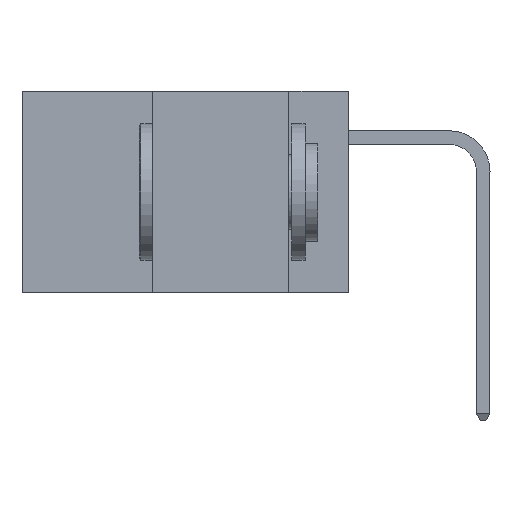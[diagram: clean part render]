
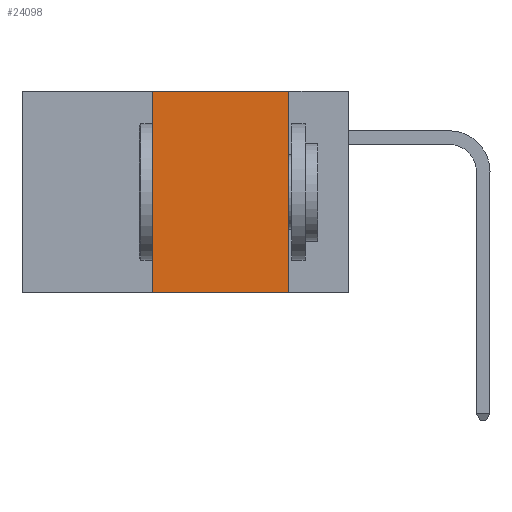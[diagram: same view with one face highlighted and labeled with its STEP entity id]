
A CAD part, left-side view. The second image highlights one B-rep face of the part: STEP entity #24098.
In plain terms, the highlighted planar face has unit normal (-1, 0, 0).
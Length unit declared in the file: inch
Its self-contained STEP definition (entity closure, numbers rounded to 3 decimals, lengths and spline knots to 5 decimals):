
#1826 = EDGE_CURVE ( 'NONE', #2224, #15288, #28103, .T. ) ;
#2224 = VERTEX_POINT ( 'NONE', #34427 ) ;
#2913 = VECTOR ( 'NONE', #7271, 39.37008 ) ;
#3601 = CARTESIAN_POINT ( 'NONE',  ( 0., 0.36, 0. ) ) ;
#5559 = EDGE_LOOP ( 'NONE', ( #30382, #32151, #26294, #21564 ) ) ;
#6026 = DIRECTION ( 'NONE',  ( 0., 0., -1. ) ) ;
#7073 = LINE ( 'NONE', #3601, #22240 ) ;
#7271 = DIRECTION ( 'NONE',  ( 0., -1., 0. ) ) ;
#11660 = LINE ( 'NONE', #21625, #2913 ) ;
#12340 = DIRECTION ( 'NONE',  ( 0., 0., 1. ) ) ;
#12544 = EDGE_CURVE ( 'NONE', #22524, #2224, #23413, .T. ) ;
#13331 = AXIS2_PLACEMENT_3D ( 'NONE', #20312, #23101, #6026 ) ;
#15288 = VERTEX_POINT ( 'NONE', #19332 ) ;
#16346 = EDGE_CURVE ( 'NONE', #26613, #15288, #11660, .T. ) ;
#18051 = DIRECTION ( 'NONE',  ( 0., -1., 0. ) ) ;
#19332 = CARTESIAN_POINT ( 'NONE',  ( 0., 0.11, -0.37 ) ) ;
#20312 = CARTESIAN_POINT ( 'NONE',  ( 0., 0.6, 0. ) ) ;
#21564 = ORIENTED_EDGE ( 'NONE', *, *, #16346, .T. ) ;
#21625 = CARTESIAN_POINT ( 'NONE',  ( 0., 0.6, -0.37 ) ) ;
#21752 = CARTESIAN_POINT ( 'NONE',  ( 0., 0.11, 0. ) ) ;
#22240 = VECTOR ( 'NONE', #12340, 39.37008 ) ;
#22524 = VERTEX_POINT ( 'NONE', #33037 ) ;
#23101 = DIRECTION ( 'NONE',  ( 1., 0., 0. ) ) ;
#23413 = LINE ( 'NONE', #26504, #29990 ) ;
#24098 = ADVANCED_FACE ( 'NONE', ( #30096 ), #31378, .F. ) ;
#24328 = DIRECTION ( 'NONE',  ( 0., 0., -1. ) ) ;
#26294 = ORIENTED_EDGE ( 'NONE', *, *, #27609, .F. ) ;
#26504 = CARTESIAN_POINT ( 'NONE',  ( 0., 0.6, 0. ) ) ;
#26613 = VERTEX_POINT ( 'NONE', #27316 ) ;
#27316 = CARTESIAN_POINT ( 'NONE',  ( 0., 0.36, -0.37 ) ) ;
#27609 = EDGE_CURVE ( 'NONE', #26613, #22524, #7073, .T. ) ;
#28103 = LINE ( 'NONE', #21752, #28976 ) ;
#28976 = VECTOR ( 'NONE', #24328, 39.37008 ) ;
#29990 = VECTOR ( 'NONE', #18051, 39.37008 ) ;
#30096 = FACE_OUTER_BOUND ( 'NONE', #5559, .T. ) ;
#30382 = ORIENTED_EDGE ( 'NONE', *, *, #1826, .F. ) ;
#31378 = PLANE ( 'NONE',  #13331 ) ;
#32151 = ORIENTED_EDGE ( 'NONE', *, *, #12544, .F. ) ;
#33037 = CARTESIAN_POINT ( 'NONE',  ( 0., 0.36, 0. ) ) ;
#34427 = CARTESIAN_POINT ( 'NONE',  ( 0., 0.11, 0. ) ) ;
